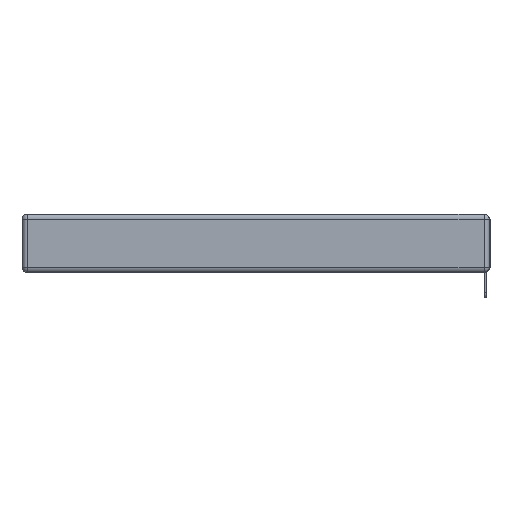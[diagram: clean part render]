
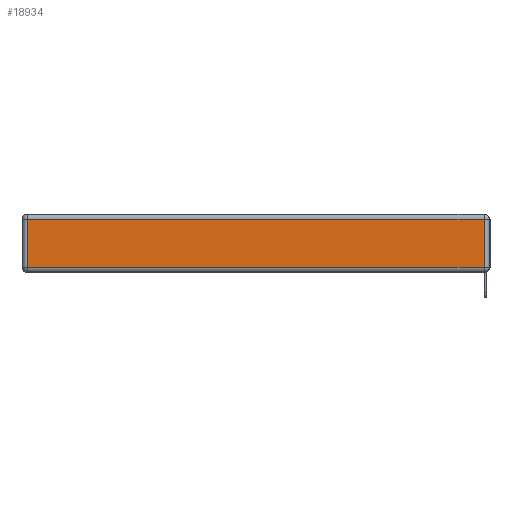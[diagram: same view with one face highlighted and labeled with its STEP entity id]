
A CAD part, left-side view. The second image highlights one B-rep face of the part: STEP entity #18934.
In plain terms, the highlighted planar face has unit normal (-1, 0, 0).
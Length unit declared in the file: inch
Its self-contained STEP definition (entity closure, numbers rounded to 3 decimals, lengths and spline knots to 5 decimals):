
#362 = CARTESIAN_POINT ( 'NONE',  ( 0., 0., -0.343 ) ) ;
#459 = FACE_OUTER_BOUND ( 'NONE', #12522, .T. ) ;
#747 = DIRECTION ( 'NONE',  ( 0., -1., 0. ) ) ;
#1106 = VECTOR ( 'NONE', #14168, 39.37008 ) ;
#1526 = VERTEX_POINT ( 'NONE', #17860 ) ;
#1572 = VERTEX_POINT ( 'NONE', #4920 ) ;
#1758 = ORIENTED_EDGE ( 'NONE', *, *, #2071, .T. ) ;
#1893 = VERTEX_POINT ( 'NONE', #15281 ) ;
#2071 = EDGE_CURVE ( 'NONE', #1526, #1893, #12848, .T. ) ;
#2336 = CARTESIAN_POINT ( 'NONE',  ( 0., 2.72, -0.343 ) ) ;
#2351 = CARTESIAN_POINT ( 'NONE',  ( 0., 0.03, -0.343 ) ) ;
#2582 = CARTESIAN_POINT ( 'NONE',  ( 0., 0., -0.313 ) ) ;
#2737 = LINE ( 'NONE', #2351, #17364 ) ;
#2926 = CARTESIAN_POINT ( 'NONE',  ( 0., 2.75, -0.03 ) ) ;
#3998 = DIRECTION ( 'NONE',  ( 0., 1., 0. ) ) ;
#4920 = CARTESIAN_POINT ( 'NONE',  ( 0., 2.72, -0.03 ) ) ;
#5781 = VECTOR ( 'NONE', #3998, 39.37008 ) ;
#7067 = EDGE_CURVE ( 'NONE', #1572, #1526, #9607, .T. ) ;
#8272 = DIRECTION ( 'NONE',  ( 0., 0., 1. ) ) ;
#9607 = LINE ( 'NONE', #2336, #1106 ) ;
#10186 = ORIENTED_EDGE ( 'NONE', *, *, #10397, .T. ) ;
#10397 = EDGE_CURVE ( 'NONE', #14273, #1572, #16226, .T. ) ;
#10450 = DIRECTION ( 'NONE',  ( -1., 0., 0. ) ) ;
#10549 = DIRECTION ( 'NONE',  ( 0., 0., 1. ) ) ;
#10931 = ORIENTED_EDGE ( 'NONE', *, *, #14792, .T. ) ;
#11189 = AXIS2_PLACEMENT_3D ( 'NONE', #362, #10450, #10549 ) ;
#12522 = EDGE_LOOP ( 'NONE', ( #1758, #10931, #10186, #13692 ) ) ;
#12848 = LINE ( 'NONE', #2582, #15537 ) ;
#13692 = ORIENTED_EDGE ( 'NONE', *, *, #7067, .T. ) ;
#14168 = DIRECTION ( 'NONE',  ( 0., 0., -1. ) ) ;
#14273 = VERTEX_POINT ( 'NONE', #15955 ) ;
#14792 = EDGE_CURVE ( 'NONE', #1893, #14273, #2737, .T. ) ;
#15281 = CARTESIAN_POINT ( 'NONE',  ( 0., 0.03, -0.313 ) ) ;
#15537 = VECTOR ( 'NONE', #747, 39.37008 ) ;
#15955 = CARTESIAN_POINT ( 'NONE',  ( 0., 0.03, -0.03 ) ) ;
#16226 = LINE ( 'NONE', #2926, #5781 ) ;
#16468 = PLANE ( 'NONE',  #11189 ) ;
#17364 = VECTOR ( 'NONE', #8272, 39.37008 ) ;
#17860 = CARTESIAN_POINT ( 'NONE',  ( 0., 2.72, -0.313 ) ) ;
#18934 = ADVANCED_FACE ( 'NONE', ( #459 ), #16468, .T. ) ;
